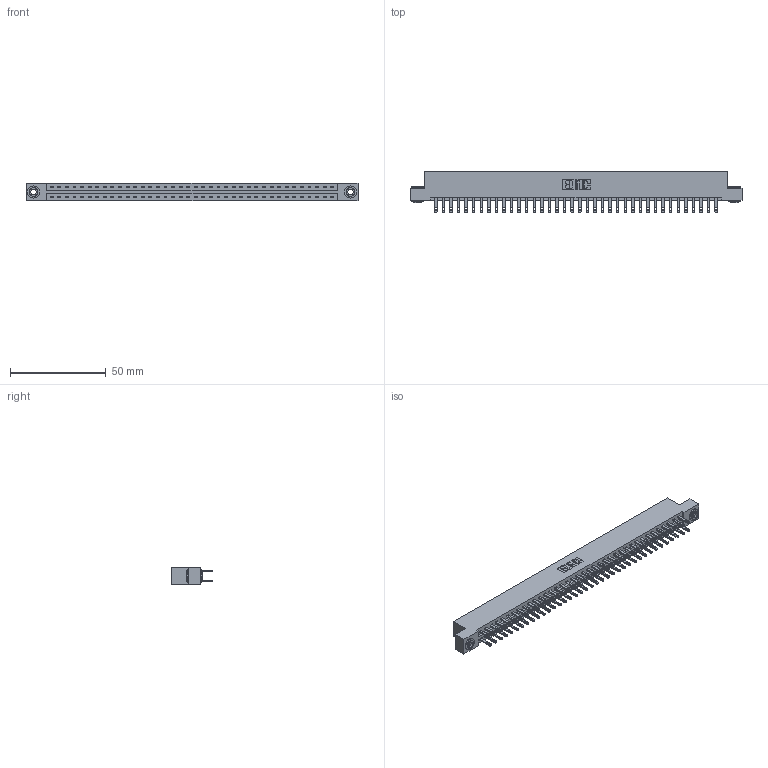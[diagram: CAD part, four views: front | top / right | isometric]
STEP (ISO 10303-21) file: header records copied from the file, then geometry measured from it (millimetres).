
FILE_DESCRIPTION (( 'STEP AP203' ), '1' );
FILE_NAME ('337-076-500-203.STEP', '2018-08-11T19:01:17', ( '' ), ( '' ), 'SwSTEP 2.0', 'SolidWorks 2016', '' );
FILE_SCHEMA (( 'CONFIG_CONTROL_DESIGN' ));
Length unit declared in the file: inch
Products named in the file (4): 337-076-500-203; 337 Part_Flush Mounting Lugs - 0.156 Dia-TH; 345-292-001_345-293-100; 345-250-002_345-250-002-102
Assembly tree (79 placements, depth 2):
  337-076-500-203
    337 Part_Flush Mounting Lugs - 0.156 Dia-TH
    345-292-001_345-293-100  x76
    345-250-002_345-250-002-102  x2
Bounding box: 173.58 x 21.85 x 9.4 mm (x, y, z)
Volume: 18492 mm3; surface area: 21934.1 mm2
Topology: 79 solids, 79 shells, 3952 faces, 12015 edges, 8006 vertices
Faces by surface type: plane 2512, cylinder 1432, cone 8
Entity records: 30560 total; most frequent: CARTESIAN_POINT 5125, ORIENTED_EDGE 5054, DIRECTION 4401, EDGE_CURVE 2527, LINE 2371, VECTOR 2371, VERTEX_POINT 1682, AXIS2_PLACEMENT_3D 1015
